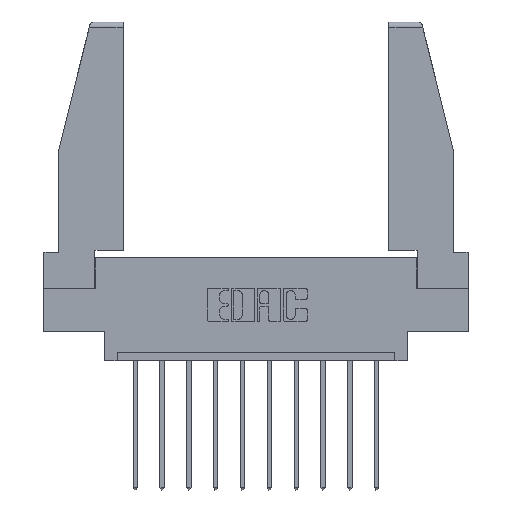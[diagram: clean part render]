
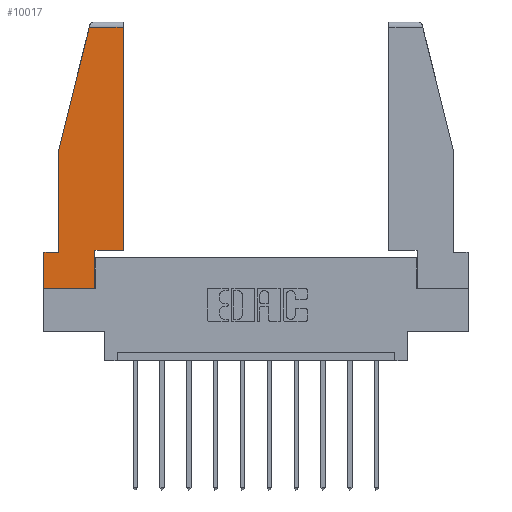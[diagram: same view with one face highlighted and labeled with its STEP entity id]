
A CAD part, top view. The second image highlights one B-rep face of the part: STEP entity #10017.
In plain terms, the highlighted planar face has unit normal (0, 0, 1).
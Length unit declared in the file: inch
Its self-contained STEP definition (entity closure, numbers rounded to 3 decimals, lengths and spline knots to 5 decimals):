
#107 = VERTEX_POINT ( 'NONE', #6926 ) ;
#335 = DIRECTION ( 'NONE',  ( 0., -1., 0. ) ) ;
#345 = CARTESIAN_POINT ( 'NONE',  ( 0., 0.21, 0. ) ) ;
#1232 = DIRECTION ( 'NONE',  ( 1., 0., 0. ) ) ;
#1622 = PLANE ( 'NONE',  #10730 ) ;
#1878 = LINE ( 'NONE', #11077, #7658 ) ;
#1941 = DIRECTION ( 'NONE',  ( -0.239, -0.971, 0. ) ) ;
#2140 = CARTESIAN_POINT ( 'NONE',  ( 0.297, 0.223, 0. ) ) ;
#2377 = CARTESIAN_POINT ( 'NONE',  ( 0., 0., 0. ) ) ;
#2511 = DIRECTION ( 'NONE',  ( -1., 0., 0. ) ) ;
#2542 = LINE ( 'NONE', #4404, #12831 ) ;
#2579 = ORIENTED_EDGE ( 'NONE', *, *, #12179, .T. ) ;
#3022 = ORIENTED_EDGE ( 'NONE', *, *, #10712, .T. ) ;
#3177 = ORIENTED_EDGE ( 'NONE', *, *, #10444, .T. ) ;
#3226 = EDGE_CURVE ( 'NONE', #7119, #9118, #6674, .T. ) ;
#3240 = CARTESIAN_POINT ( 'NONE',  ( 0., 0., 0. ) ) ;
#3291 = VERTEX_POINT ( 'NONE', #9103 ) ;
#3780 = DIRECTION ( 'NONE',  ( 1., 0., 0. ) ) ;
#3948 = LINE ( 'NONE', #13987, #10820 ) ;
#4052 = EDGE_CURVE ( 'NONE', #6053, #11730, #1878, .T. ) ;
#4289 = VERTEX_POINT ( 'NONE', #12209 ) ;
#4404 = CARTESIAN_POINT ( 'NONE',  ( 0.297, 0., 0. ) ) ;
#5346 = ORIENTED_EDGE ( 'NONE', *, *, #13048, .T. ) ;
#5429 = VERTEX_POINT ( 'NONE', #8162 ) ;
#6053 = VERTEX_POINT ( 'NONE', #10607 ) ;
#6319 = VECTOR ( 'NONE', #335, 39.37008 ) ;
#6574 = CARTESIAN_POINT ( 'NONE',  ( 0., 1.52, 0. ) ) ;
#6660 = VECTOR ( 'NONE', #2511, 39.37008 ) ;
#6674 = LINE ( 'NONE', #11284, #6996 ) ;
#6825 = DIRECTION ( 'NONE',  ( -1., 0., 0. ) ) ;
#6926 = CARTESIAN_POINT ( 'NONE',  ( 0.2636, 1.52, 0. ) ) ;
#6941 = VECTOR ( 'NONE', #7472, 39.37008 ) ;
#6962 = ORIENTED_EDGE ( 'NONE', *, *, #9791, .T. ) ;
#6970 = ORIENTED_EDGE ( 'NONE', *, *, #9053, .T. ) ;
#6996 = VECTOR ( 'NONE', #12132, 39.37008 ) ;
#7119 = VERTEX_POINT ( 'NONE', #8034 ) ;
#7154 = ORIENTED_EDGE ( 'NONE', *, *, #11782, .T. ) ;
#7212 = VERTEX_POINT ( 'NONE', #10803 ) ;
#7296 = LINE ( 'NONE', #3240, #6941 ) ;
#7360 = CARTESIAN_POINT ( 'NONE',  ( 0.461, 1.52, 0. ) ) ;
#7472 = DIRECTION ( 'NONE',  ( 1., 0., 0. ) ) ;
#7658 = VECTOR ( 'NONE', #7718, 39.37008 ) ;
#7718 = DIRECTION ( 'NONE',  ( 0., 1., 0. ) ) ;
#8034 = CARTESIAN_POINT ( 'NONE',  ( 0., 0.21, 0. ) ) ;
#8162 = CARTESIAN_POINT ( 'NONE',  ( 0.297, 0.223, 0. ) ) ;
#8175 = CARTESIAN_POINT ( 'NONE',  ( 0., 0., 0. ) ) ;
#9053 = EDGE_CURVE ( 'NONE', #3291, #5429, #2542, .T. ) ;
#9082 = CARTESIAN_POINT ( 'NONE',  ( 0.086, 0.8, 0. ) ) ;
#9103 = CARTESIAN_POINT ( 'NONE',  ( 0.297, 0., 0. ) ) ;
#9118 = VERTEX_POINT ( 'NONE', #2377 ) ;
#9200 = LINE ( 'NONE', #345, #6660 ) ;
#9227 = DIRECTION ( 'NONE',  ( 0., 0., 1. ) ) ;
#9369 = ORIENTED_EDGE ( 'NONE', *, *, #3226, .T. ) ;
#9557 = DIRECTION ( 'NONE',  ( 0., 1., 0. ) ) ;
#9791 = EDGE_CURVE ( 'NONE', #7212, #4289, #11078, .T. ) ;
#10017 = ADVANCED_FACE ( 'NONE', ( #13137 ), #1622, .T. ) ;
#10117 = ORIENTED_EDGE ( 'NONE', *, *, #4052, .T. ) ;
#10198 = VECTOR ( 'NONE', #6825, 39.37008 ) ;
#10444 = EDGE_CURVE ( 'NONE', #11730, #107, #13119, .T. ) ;
#10607 = CARTESIAN_POINT ( 'NONE',  ( 0.461, 0.223, 0. ) ) ;
#10635 = EDGE_LOOP ( 'NONE', ( #10117, #3177, #3022, #6962, #7154, #9369, #5346, #6970, #2579 ) ) ;
#10712 = EDGE_CURVE ( 'NONE', #107, #7212, #3948, .T. ) ;
#10730 = AXIS2_PLACEMENT_3D ( 'NONE', #8175, #9227, #3780 ) ;
#10803 = CARTESIAN_POINT ( 'NONE',  ( 0.086, 0.8, 0. ) ) ;
#10820 = VECTOR ( 'NONE', #1941, 39.37008 ) ;
#11077 = CARTESIAN_POINT ( 'NONE',  ( 0.461, 0.223, 0. ) ) ;
#11078 = LINE ( 'NONE', #9082, #6319 ) ;
#11284 = CARTESIAN_POINT ( 'NONE',  ( 0., 0.21, 0. ) ) ;
#11433 = VECTOR ( 'NONE', #1232, 39.37008 ) ;
#11730 = VERTEX_POINT ( 'NONE', #7360 ) ;
#11782 = EDGE_CURVE ( 'NONE', #4289, #7119, #9200, .T. ) ;
#11950 = LINE ( 'NONE', #2140, #11433 ) ;
#12132 = DIRECTION ( 'NONE',  ( 0., -1., 0. ) ) ;
#12179 = EDGE_CURVE ( 'NONE', #5429, #6053, #11950, .T. ) ;
#12209 = CARTESIAN_POINT ( 'NONE',  ( 0.086, 0.21, 0. ) ) ;
#12831 = VECTOR ( 'NONE', #9557, 39.37008 ) ;
#13048 = EDGE_CURVE ( 'NONE', #9118, #3291, #7296, .T. ) ;
#13119 = LINE ( 'NONE', #6574, #10198 ) ;
#13137 = FACE_OUTER_BOUND ( 'NONE', #10635, .T. ) ;
#13987 = CARTESIAN_POINT ( 'NONE',  ( 0.271, 1.55, 0. ) ) ;
